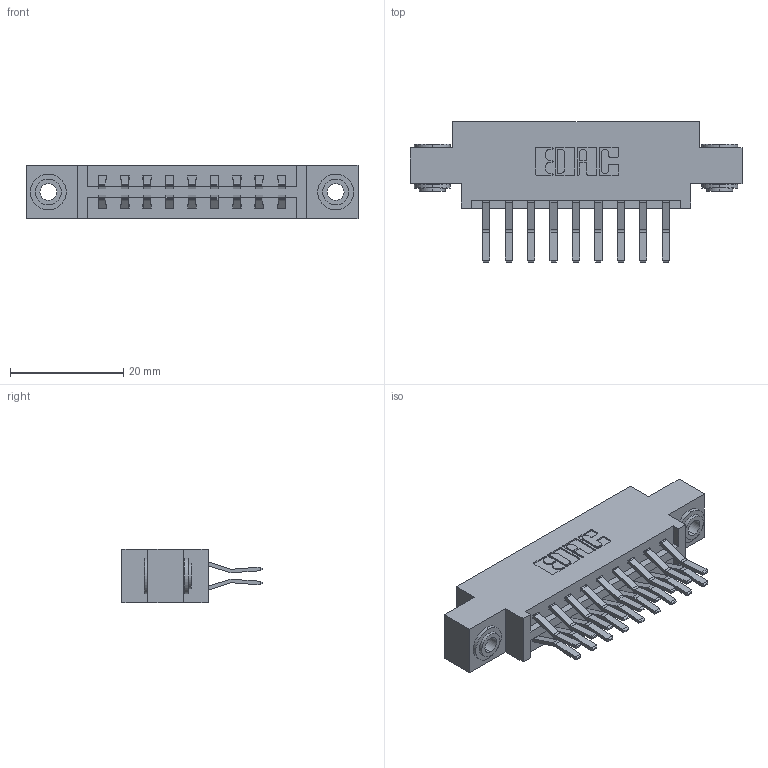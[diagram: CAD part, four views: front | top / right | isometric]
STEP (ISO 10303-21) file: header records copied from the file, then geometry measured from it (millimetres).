
FILE_DESCRIPTION (( 'STEP AP203' ), '1' );
FILE_NAME ('337-018-560-803.STEP', '2019-10-10T19:03:27', ( '' ), ( '' ), 'SwSTEP 2.0', 'SolidWorks 2016', '' );
FILE_SCHEMA (( 'CONFIG_CONTROL_DESIGN' ));
Length unit declared in the file: inch
Products named in the file (4): 345-292-001_560 Tail; 337 Part_0.170 Offset - 0.156 Dia-TH; 345-250-002_345-250-002-102; 337-018-560-803
Assembly tree (21 placements, depth 2):
  337-018-560-803
    337 Part_0.170 Offset - 0.156 Dia-TH
    345-292-001_560 Tail  x18
    345-250-002_345-250-002-102  x2
Bounding box: 58.67 x 24.78 x 9.4 mm (x, y, z)
Volume: 5764.1 mm3; surface area: 6869.5 mm2
Topology: 21 solids, 21 shells, 1164 faces, 3405 edges, 2242 vertices
Faces by surface type: plane 768, cylinder 388, cone 8
Entity records: 12116 total; most frequent: CARTESIAN_POINT 2045, ORIENTED_EDGE 1974, DIRECTION 1837, EDGE_CURVE 987, VECTOR 831, LINE 831, VERTEX_POINT 654, AXIS2_PLACEMENT_3D 503
